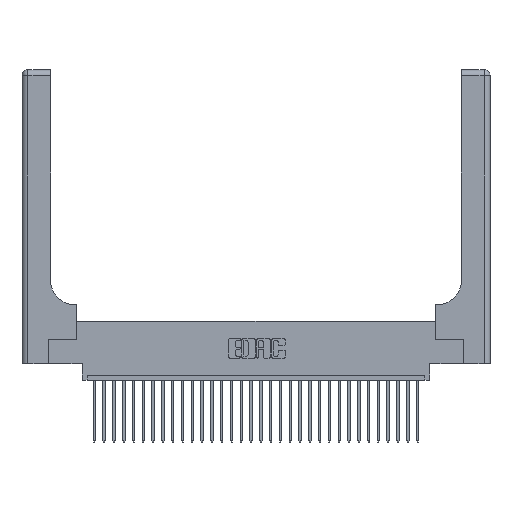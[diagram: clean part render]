
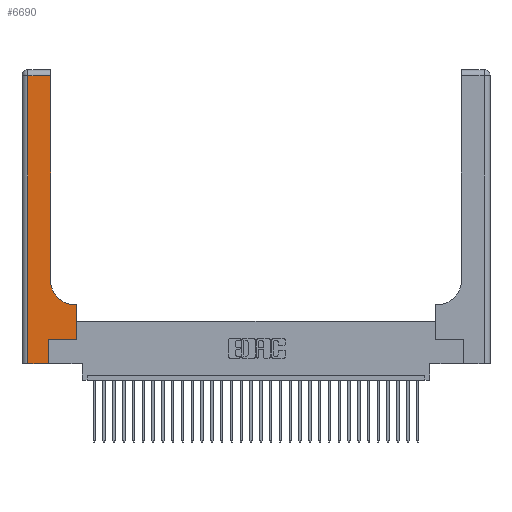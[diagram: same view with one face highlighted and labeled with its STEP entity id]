
A CAD part, top view. The second image highlights one B-rep face of the part: STEP entity #6690.
In plain terms, the highlighted planar face has unit normal (0, 0, 1).
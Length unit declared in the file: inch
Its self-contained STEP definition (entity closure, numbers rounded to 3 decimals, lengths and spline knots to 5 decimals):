
#586 = DIRECTION ( 'NONE',  ( 0., 1., 0. ) ) ;
#1004 = ORIENTED_EDGE ( 'NONE', *, *, #23734, .T. ) ;
#1484 = VERTEX_POINT ( 'NONE', #22256 ) ;
#2210 = CARTESIAN_POINT ( 'NONE',  ( 0.2915, 0.6, 0.37 ) ) ;
#2265 = VECTOR ( 'NONE', #7335, 39.37008 ) ;
#2294 = VERTEX_POINT ( 'NONE', #30592 ) ;
#2373 = ORIENTED_EDGE ( 'NONE', *, *, #3546, .T. ) ;
#2565 = CARTESIAN_POINT ( 'NONE',  ( 0.269, 0., 0.37 ) ) ;
#2819 = DIRECTION ( 'NONE',  ( 1., 0., 0. ) ) ;
#3087 = VECTOR ( 'NONE', #2819, 39.37008 ) ;
#3546 = EDGE_CURVE ( 'NONE', #23531, #2294, #8489, .T. ) ;
#3640 = AXIS2_PLACEMENT_3D ( 'NONE', #11913, #16676, #13973 ) ;
#3712 = VERTEX_POINT ( 'NONE', #5034 ) ;
#3795 = VERTEX_POINT ( 'NONE', #25772 ) ;
#4655 = EDGE_CURVE ( 'NONE', #20670, #3712, #6269, .T. ) ;
#5034 = CARTESIAN_POINT ( 'NONE',  ( 0.5415, 0.6, 0.37 ) ) ;
#5153 = DIRECTION ( 'NONE',  ( -1., 0., 0. ) ) ;
#6269 = LINE ( 'NONE', #2210, #31764 ) ;
#6351 = DIRECTION ( 'NONE',  ( 1., 0., 0. ) ) ;
#6491 = ORIENTED_EDGE ( 'NONE', *, *, #23130, .T. ) ;
#6690 = ADVANCED_FACE ( 'NONE', ( #30850 ), #26450, .F. ) ;
#7335 = DIRECTION ( 'NONE',  ( 0., -1., 0. ) ) ;
#7569 = CARTESIAN_POINT ( 'NONE',  ( 0.5585, 0.6, 0.37 ) ) ;
#7654 = VECTOR ( 'NONE', #13022, 39.37008 ) ;
#7958 = CARTESIAN_POINT ( 'NONE',  ( 0.269, 0.25, 0.37 ) ) ;
#8489 = LINE ( 'NONE', #2565, #22369 ) ;
#8571 = EDGE_CURVE ( 'NONE', #3712, #15832, #14897, .T. ) ;
#9182 = LINE ( 'NONE', #7958, #7654 ) ;
#10073 = DIRECTION ( 'NONE',  ( 0., 1., 0. ) ) ;
#10308 = VECTOR ( 'NONE', #5153, 39.37008 ) ;
#11664 = ORIENTED_EDGE ( 'NONE', *, *, #16161, .T. ) ;
#11913 = CARTESIAN_POINT ( 'NONE',  ( 0., 3., 0.37 ) ) ;
#13022 = DIRECTION ( 'NONE',  ( 1., 0., 0. ) ) ;
#13137 = CARTESIAN_POINT ( 'NONE',  ( 0.2915, 0.85, 0.37 ) ) ;
#13953 = EDGE_LOOP ( 'NONE', ( #14902, #1004, #11664, #18114, #2373, #6491, #18379, #15851, #26110 ) ) ;
#13973 = DIRECTION ( 'NONE',  ( -1., 0., 0. ) ) ;
#14621 = VERTEX_POINT ( 'NONE', #22990 ) ;
#14897 = CIRCLE ( 'NONE', #29093, 0.25 ) ;
#14902 = ORIENTED_EDGE ( 'NONE', *, *, #27556, .T. ) ;
#15613 = EDGE_CURVE ( 'NONE', #3795, #23531, #23067, .T. ) ;
#15832 = VERTEX_POINT ( 'NONE', #13137 ) ;
#15851 = ORIENTED_EDGE ( 'NONE', *, *, #4655, .T. ) ;
#16161 = EDGE_CURVE ( 'NONE', #27965, #3795, #22681, .T. ) ;
#16654 = LINE ( 'NONE', #20838, #30539 ) ;
#16676 = DIRECTION ( 'NONE',  ( 0., 0., -1. ) ) ;
#17936 = DIRECTION ( 'NONE',  ( 0., 1., 0. ) ) ;
#18114 = ORIENTED_EDGE ( 'NONE', *, *, #15613, .T. ) ;
#18379 = ORIENTED_EDGE ( 'NONE', *, *, #19403, .T. ) ;
#19348 = LINE ( 'NONE', #19770, #20515 ) ;
#19403 = EDGE_CURVE ( 'NONE', #14621, #20670, #19348, .T. ) ;
#19491 = CARTESIAN_POINT ( 'NONE',  ( 0.06, 3., 0.37 ) ) ;
#19770 = CARTESIAN_POINT ( 'NONE',  ( 0.5585, 0.25, 0.37 ) ) ;
#20343 = LINE ( 'NONE', #22349, #10308 ) ;
#20515 = VECTOR ( 'NONE', #10073, 39.37008 ) ;
#20670 = VERTEX_POINT ( 'NONE', #7569 ) ;
#20838 = CARTESIAN_POINT ( 'NONE',  ( 0.2915, 3., 0.37 ) ) ;
#21718 = CARTESIAN_POINT ( 'NONE',  ( 0.269, 0., 0.37 ) ) ;
#21819 = DIRECTION ( 'NONE',  ( -1., 0., 0. ) ) ;
#22256 = CARTESIAN_POINT ( 'NONE',  ( 0.2915, 2.94, 0.37 ) ) ;
#22349 = CARTESIAN_POINT ( 'NONE',  ( 0., 2.94, 0.37 ) ) ;
#22369 = VECTOR ( 'NONE', #586, 39.37008 ) ;
#22681 = LINE ( 'NONE', #19491, #2265 ) ;
#22990 = CARTESIAN_POINT ( 'NONE',  ( 0.5585, 0.25, 0.37 ) ) ;
#23067 = LINE ( 'NONE', #24862, #3087 ) ;
#23130 = EDGE_CURVE ( 'NONE', #2294, #14621, #9182, .T. ) ;
#23336 = DIRECTION ( 'NONE',  ( 0., 0., -1. ) ) ;
#23531 = VERTEX_POINT ( 'NONE', #21718 ) ;
#23647 = CARTESIAN_POINT ( 'NONE',  ( 0.5415, 0.85, 0.37 ) ) ;
#23734 = EDGE_CURVE ( 'NONE', #1484, #27965, #20343, .T. ) ;
#24862 = CARTESIAN_POINT ( 'NONE',  ( 0., 0., 0.37 ) ) ;
#25772 = CARTESIAN_POINT ( 'NONE',  ( 0.06, 0., 0.37 ) ) ;
#26110 = ORIENTED_EDGE ( 'NONE', *, *, #8571, .T. ) ;
#26450 = PLANE ( 'NONE',  #3640 ) ;
#27556 = EDGE_CURVE ( 'NONE', #15832, #1484, #16654, .T. ) ;
#27965 = VERTEX_POINT ( 'NONE', #31441 ) ;
#29093 = AXIS2_PLACEMENT_3D ( 'NONE', #23647, #23336, #6351 ) ;
#30539 = VECTOR ( 'NONE', #17936, 39.37008 ) ;
#30592 = CARTESIAN_POINT ( 'NONE',  ( 0.269, 0.25, 0.37 ) ) ;
#30850 = FACE_OUTER_BOUND ( 'NONE', #13953, .T. ) ;
#31441 = CARTESIAN_POINT ( 'NONE',  ( 0.06, 2.94, 0.37 ) ) ;
#31764 = VECTOR ( 'NONE', #21819, 39.37008 ) ;
